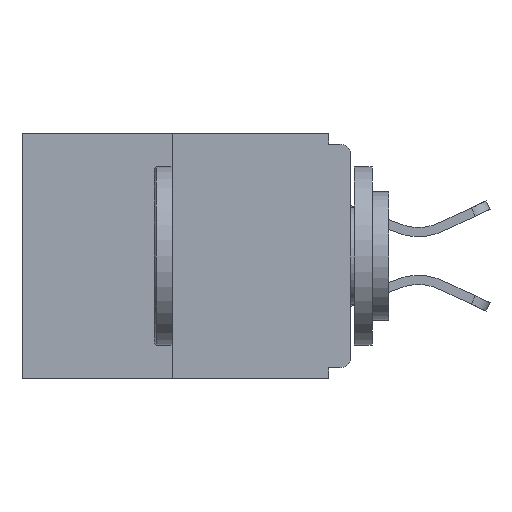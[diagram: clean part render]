
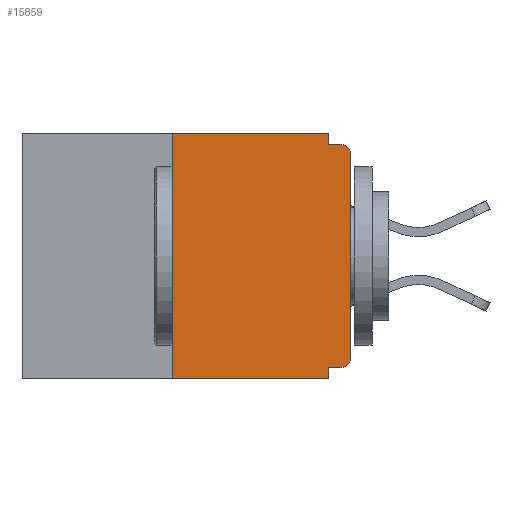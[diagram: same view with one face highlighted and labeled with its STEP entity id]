
A CAD part, left-side view. The second image highlights one B-rep face of the part: STEP entity #15859.
In plain terms, the highlighted planar face has unit normal (-1, 0, 0).
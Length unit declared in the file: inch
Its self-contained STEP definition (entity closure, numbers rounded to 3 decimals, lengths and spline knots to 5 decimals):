
#1228 = DIRECTION ( 'NONE',  ( 0., 0., 1. ) ) ;
#1256 = ORIENTED_EDGE ( 'NONE', *, *, #13647, .F. ) ;
#1381 = CARTESIAN_POINT ( 'NONE',  ( 0., 0.031, -0.343 ) ) ;
#1554 = EDGE_CURVE ( 'NONE', #2148, #16165, #20153, .T. ) ;
#1564 = DIRECTION ( 'NONE',  ( 0., -1., 0. ) ) ;
#1571 = CARTESIAN_POINT ( 'NONE',  ( 0., 0.25, 0. ) ) ;
#2015 = VERTEX_POINT ( 'NONE', #6805 ) ;
#2148 = VERTEX_POINT ( 'NONE', #10650 ) ;
#2278 = EDGE_LOOP ( 'NONE', ( #22144, #1256, #9746, #19124, #18089, #20600, #17113, #24990, #16337, #7105 ) ) ;
#3269 = VECTOR ( 'NONE', #23567, 39.37008 ) ;
#4199 = EDGE_CURVE ( 'NONE', #9401, #13732, #10041, .T. ) ;
#5055 = DIRECTION ( 'NONE',  ( 0., -1., 0. ) ) ;
#5435 = DIRECTION ( 'NONE',  ( -1., 0., 0. ) ) ;
#5563 = CARTESIAN_POINT ( 'NONE',  ( 0., 0.46, 0. ) ) ;
#5649 = VERTEX_POINT ( 'NONE', #1571 ) ;
#5659 = PLANE ( 'NONE',  #9494 ) ;
#5837 = LINE ( 'NONE', #17637, #16720 ) ;
#5878 = FACE_OUTER_BOUND ( 'NONE', #2278, .T. ) ;
#6036 = CARTESIAN_POINT ( 'NONE',  ( 0., 0.031, -0.343 ) ) ;
#6805 = CARTESIAN_POINT ( 'NONE',  ( 0., 0.031, -0.328 ) ) ;
#7065 = LINE ( 'NONE', #14189, #15323 ) ;
#7105 = ORIENTED_EDGE ( 'NONE', *, *, #1554, .F. ) ;
#7462 = VERTEX_POINT ( 'NONE', #17654 ) ;
#7490 = CARTESIAN_POINT ( 'NONE',  ( 0., 0.46, 0. ) ) ;
#7580 = DIRECTION ( 'NONE',  ( 0., 0., -1. ) ) ;
#7760 = VERTEX_POINT ( 'NONE', #14239 ) ;
#7898 = LINE ( 'NONE', #26690, #16830 ) ;
#9401 = VERTEX_POINT ( 'NONE', #10576 ) ;
#9494 = AXIS2_PLACEMENT_3D ( 'NONE', #5563, #11956, #16385 ) ;
#9518 = CARTESIAN_POINT ( 'NONE',  ( 0., 0.031, -0.015 ) ) ;
#9746 = ORIENTED_EDGE ( 'NONE', *, *, #16041, .T. ) ;
#10041 = CIRCLE ( 'NONE', #18744, 0.015 ) ;
#10164 = EDGE_CURVE ( 'NONE', #2015, #14716, #18000, .T. ) ;
#10576 = CARTESIAN_POINT ( 'NONE',  ( 0., 0.015, -0.328 ) ) ;
#10650 = CARTESIAN_POINT ( 'NONE',  ( 0., 0.031, 0. ) ) ;
#10731 = EDGE_CURVE ( 'NONE', #9401, #2015, #5837, .T. ) ;
#10758 = CIRCLE ( 'NONE', #26252, 0.015 ) ;
#11849 = DIRECTION ( 'NONE',  ( 0., 0., -1. ) ) ;
#11956 = DIRECTION ( 'NONE',  ( 1., 0., 0. ) ) ;
#12047 = CARTESIAN_POINT ( 'NONE',  ( 0., 0.015, -0.313 ) ) ;
#12591 = VECTOR ( 'NONE', #22677, 39.37008 ) ;
#13048 = LINE ( 'NONE', #7490, #23644 ) ;
#13647 = EDGE_CURVE ( 'NONE', #14669, #5649, #20512, .T. ) ;
#13732 = VERTEX_POINT ( 'NONE', #17275 ) ;
#13741 = CARTESIAN_POINT ( 'NONE',  ( 0., 0.25, -0.343 ) ) ;
#14189 = CARTESIAN_POINT ( 'NONE',  ( 0., 0., -0.015 ) ) ;
#14239 = CARTESIAN_POINT ( 'NONE',  ( 0., 0., -0.03 ) ) ;
#14669 = VERTEX_POINT ( 'NONE', #13741 ) ;
#14716 = VERTEX_POINT ( 'NONE', #1381 ) ;
#15218 = CARTESIAN_POINT ( 'NONE',  ( 0., 0.031, 0. ) ) ;
#15323 = VECTOR ( 'NONE', #1564, 39.37008 ) ;
#15350 = VECTOR ( 'NONE', #25120, 39.37008 ) ;
#15859 = ADVANCED_FACE ( 'NONE', ( #5878 ), #5659, .F. ) ;
#16041 = EDGE_CURVE ( 'NONE', #14669, #14716, #26112, .T. ) ;
#16165 = VERTEX_POINT ( 'NONE', #9518 ) ;
#16337 = ORIENTED_EDGE ( 'NONE', *, *, #26206, .F. ) ;
#16385 = DIRECTION ( 'NONE',  ( 0., 0., -1. ) ) ;
#16720 = VECTOR ( 'NONE', #26047, 39.37008 ) ;
#16830 = VECTOR ( 'NONE', #1228, 39.37008 ) ;
#17113 = ORIENTED_EDGE ( 'NONE', *, *, #25528, .T. ) ;
#17166 = EDGE_CURVE ( 'NONE', #7760, #7462, #10758, .T. ) ;
#17275 = CARTESIAN_POINT ( 'NONE',  ( 0., 0., -0.313 ) ) ;
#17637 = CARTESIAN_POINT ( 'NONE',  ( 0., 0., -0.328 ) ) ;
#17654 = CARTESIAN_POINT ( 'NONE',  ( 0., 0.015, -0.015 ) ) ;
#18000 = LINE ( 'NONE', #6036, #15350 ) ;
#18089 = ORIENTED_EDGE ( 'NONE', *, *, #10731, .F. ) ;
#18744 = AXIS2_PLACEMENT_3D ( 'NONE', #12047, #22490, #11849 ) ;
#19124 = ORIENTED_EDGE ( 'NONE', *, *, #10164, .F. ) ;
#20143 = CARTESIAN_POINT ( 'NONE',  ( 0., 0.015, -0.03 ) ) ;
#20153 = LINE ( 'NONE', #15218, #3269 ) ;
#20512 = LINE ( 'NONE', #25020, #12591 ) ;
#20600 = ORIENTED_EDGE ( 'NONE', *, *, #4199, .T. ) ;
#20921 = CARTESIAN_POINT ( 'NONE',  ( 0., 0.46, -0.343 ) ) ;
#22144 = ORIENTED_EDGE ( 'NONE', *, *, #23190, .F. ) ;
#22490 = DIRECTION ( 'NONE',  ( -1., 0., 0. ) ) ;
#22677 = DIRECTION ( 'NONE',  ( 0., 0., 1. ) ) ;
#23190 = EDGE_CURVE ( 'NONE', #5649, #2148, #13048, .T. ) ;
#23567 = DIRECTION ( 'NONE',  ( 0., 0., -1. ) ) ;
#23644 = VECTOR ( 'NONE', #5055, 39.37008 ) ;
#24400 = VECTOR ( 'NONE', #25129, 39.37008 ) ;
#24990 = ORIENTED_EDGE ( 'NONE', *, *, #17166, .T. ) ;
#25020 = CARTESIAN_POINT ( 'NONE',  ( 0., 0.25, 0. ) ) ;
#25120 = DIRECTION ( 'NONE',  ( 0., 0., -1. ) ) ;
#25129 = DIRECTION ( 'NONE',  ( 0., -1., 0. ) ) ;
#25528 = EDGE_CURVE ( 'NONE', #13732, #7760, #7898, .T. ) ;
#26047 = DIRECTION ( 'NONE',  ( 0., 1., 0. ) ) ;
#26112 = LINE ( 'NONE', #20921, #24400 ) ;
#26206 = EDGE_CURVE ( 'NONE', #16165, #7462, #7065, .T. ) ;
#26252 = AXIS2_PLACEMENT_3D ( 'NONE', #20143, #5435, #7580 ) ;
#26690 = CARTESIAN_POINT ( 'NONE',  ( 0., 0., 0. ) ) ;
